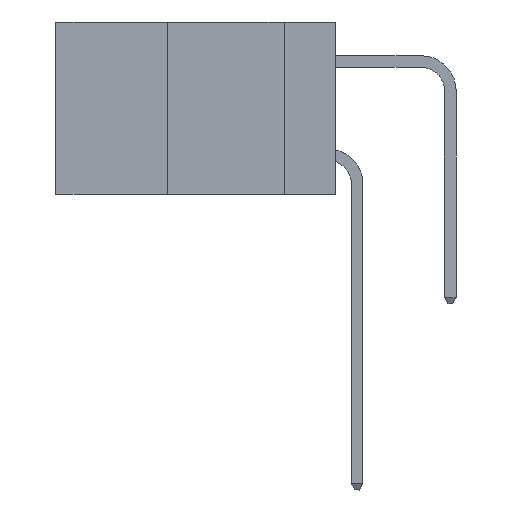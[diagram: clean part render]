
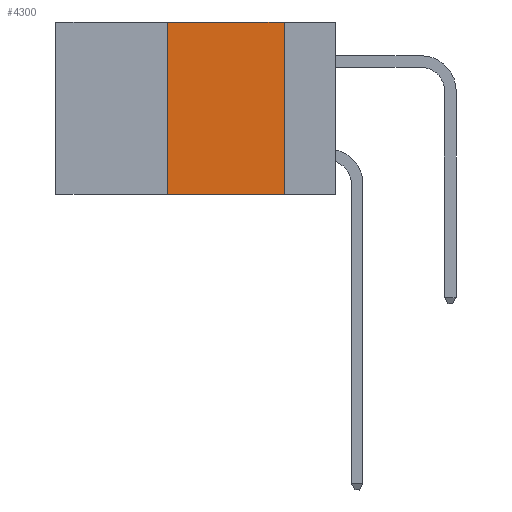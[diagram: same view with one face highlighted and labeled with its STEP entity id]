
A CAD part, left-side view. The second image highlights one B-rep face of the part: STEP entity #4300.
In plain terms, the highlighted planar face has unit normal (-1, 0, 0).
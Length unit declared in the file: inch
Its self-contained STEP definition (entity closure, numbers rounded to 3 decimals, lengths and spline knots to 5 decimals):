
#435 = LINE ( 'NONE', #4311, #14417 ) ;
#1191 = DIRECTION ( 'NONE',  ( 1., 0., 0. ) ) ;
#2766 = ORIENTED_EDGE ( 'NONE', *, *, #20435, .F. ) ;
#2867 = LINE ( 'NONE', #11325, #25305 ) ;
#3120 = CARTESIAN_POINT ( 'NONE',  ( 0., 0.6, -0.37 ) ) ;
#3248 = CARTESIAN_POINT ( 'NONE',  ( 0., 0.36, 0. ) ) ;
#4083 = VERTEX_POINT ( 'NONE', #25459 ) ;
#4200 = EDGE_CURVE ( 'NONE', #24914, #13646, #15485, .T. ) ;
#4300 = ADVANCED_FACE ( 'NONE', ( #14200 ), #20578, .F. ) ;
#4311 = CARTESIAN_POINT ( 'NONE',  ( 0., 0.11, 0. ) ) ;
#4442 = CARTESIAN_POINT ( 'NONE',  ( 0., 0.36, -0.37 ) ) ;
#5743 = DIRECTION ( 'NONE',  ( 0., 0., -1. ) ) ;
#6040 = VECTOR ( 'NONE', #17420, 39.37008 ) ;
#6534 = DIRECTION ( 'NONE',  ( 0., 0., -1. ) ) ;
#11216 = VECTOR ( 'NONE', #24322, 39.37008 ) ;
#11325 = CARTESIAN_POINT ( 'NONE',  ( 0., 0.36, 0. ) ) ;
#12421 = EDGE_LOOP ( 'NONE', ( #26688, #14452, #2766, #23573 ) ) ;
#12982 = EDGE_CURVE ( 'NONE', #25919, #4083, #15876, .T. ) ;
#13646 = VERTEX_POINT ( 'NONE', #19524 ) ;
#14200 = FACE_OUTER_BOUND ( 'NONE', #12421, .T. ) ;
#14417 = VECTOR ( 'NONE', #6534, 39.37008 ) ;
#14452 = ORIENTED_EDGE ( 'NONE', *, *, #12982, .F. ) ;
#15485 = LINE ( 'NONE', #3120, #6040 ) ;
#15811 = AXIS2_PLACEMENT_3D ( 'NONE', #27078, #1191, #5743 ) ;
#15876 = LINE ( 'NONE', #26397, #11216 ) ;
#17420 = DIRECTION ( 'NONE',  ( 0., -1., 0. ) ) ;
#19524 = CARTESIAN_POINT ( 'NONE',  ( 0., 0.11, -0.37 ) ) ;
#19772 = DIRECTION ( 'NONE',  ( 0., 0., 1. ) ) ;
#20435 = EDGE_CURVE ( 'NONE', #24914, #25919, #2867, .T. ) ;
#20578 = PLANE ( 'NONE',  #15811 ) ;
#23573 = ORIENTED_EDGE ( 'NONE', *, *, #4200, .T. ) ;
#24322 = DIRECTION ( 'NONE',  ( 0., -1., 0. ) ) ;
#24914 = VERTEX_POINT ( 'NONE', #4442 ) ;
#25305 = VECTOR ( 'NONE', #19772, 39.37008 ) ;
#25459 = CARTESIAN_POINT ( 'NONE',  ( 0., 0.11, 0. ) ) ;
#25919 = VERTEX_POINT ( 'NONE', #3248 ) ;
#26397 = CARTESIAN_POINT ( 'NONE',  ( 0., 0.6, 0. ) ) ;
#26541 = EDGE_CURVE ( 'NONE', #4083, #13646, #435, .T. ) ;
#26688 = ORIENTED_EDGE ( 'NONE', *, *, #26541, .F. ) ;
#27078 = CARTESIAN_POINT ( 'NONE',  ( 0., 0.6, 0. ) ) ;
